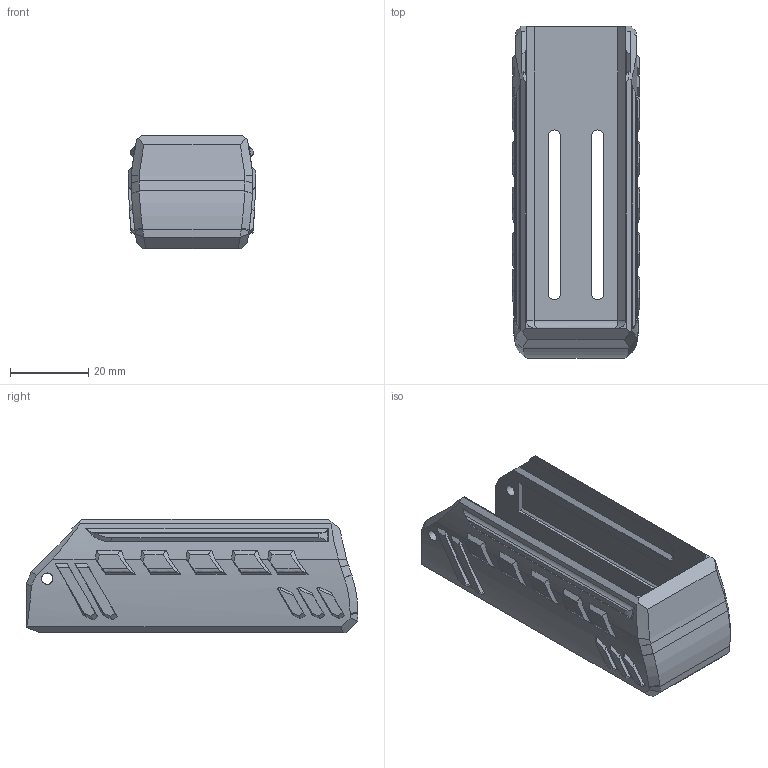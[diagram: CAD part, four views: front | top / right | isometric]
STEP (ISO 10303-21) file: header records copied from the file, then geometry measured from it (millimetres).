
FILE_DESCRIPTION(/* description */ (''),/* implementation_level */ '2;1');
FILE_NAME(/* name */ 'Slide.stp',/* time_stamp */ '2020-10-15T21:27:41-05:00',/* author */ (''),/* organization */ (''),/* preprocessor_version */ 'ST-DEVELOPER v15.2',/* originating_system */ 'Autodesk Translator Framework v2.0.0.5431',/* authorisation */ '');
FILE_SCHEMA (('AUTOMOTIVE_DESIGN { 1 0 10303 214 3 1 1 }'));
Length unit declared in the file: centimetre
Products named in the file (1): Slide
Bounding box: 32.55 x 84.6 x 29 mm (x, y, z)
Volume: 14922.2 mm3; surface area: 14651.8 mm2
Topology: 1 solids, 1 shells, 290 faces, 795 edges, 521 vertices
Faces by surface type: plane 217, bspline 42, cylinder 29, cone 2
Full cylindrical faces by diameter (mm): 2.9 x2
Entity records: 9656 total; most frequent: CARTESIAN_POINT 2470, ORIENTED_EDGE 1584, DIRECTION 1354, EDGE_CURVE 792, LINE 528, VECTOR 528, VERTEX_POINT 520, AXIS2_PLACEMENT_3D 413
